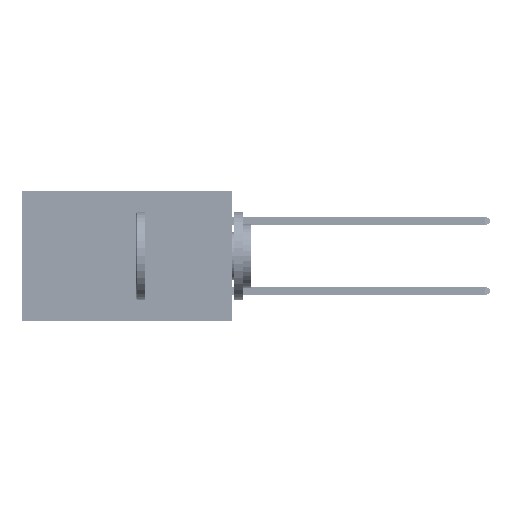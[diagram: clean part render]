
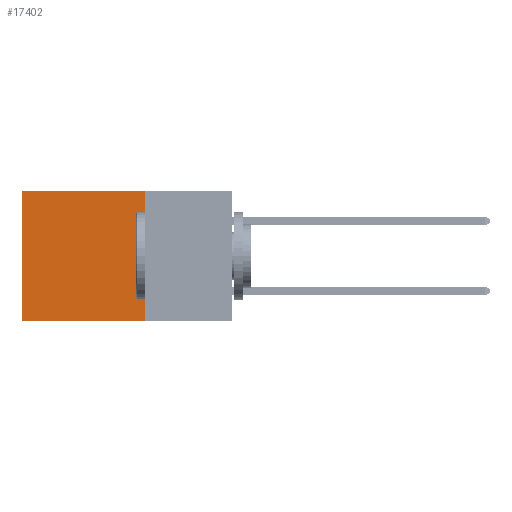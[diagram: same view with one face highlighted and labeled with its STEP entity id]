
A CAD part, left-side view. The second image highlights one B-rep face of the part: STEP entity #17402.
In plain terms, the highlighted planar face has unit normal (-1, 0, 0).
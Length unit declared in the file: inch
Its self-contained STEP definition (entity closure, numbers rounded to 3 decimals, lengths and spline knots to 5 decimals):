
#443 = VERTEX_POINT ( 'NONE', #15198 ) ;
#3101 = LINE ( 'NONE', #31345, #43478 ) ;
#3778 = EDGE_CURVE ( 'NONE', #43438, #443, #34438, .T. ) ;
#4006 = CARTESIAN_POINT ( 'NONE',  ( 0.2875, 0.25, 0. ) ) ;
#5733 = ORIENTED_EDGE ( 'NONE', *, *, #9166, .F. ) ;
#7091 = DIRECTION ( 'NONE',  ( 0., 0., -1. ) ) ;
#7413 = EDGE_LOOP ( 'NONE', ( #15483, #46881, #5733, #49461 ) ) ;
#8195 = DIRECTION ( 'NONE',  ( 0., 1., 0. ) ) ;
#8433 = FACE_OUTER_BOUND ( 'NONE', #7413, .T. ) ;
#8501 = LINE ( 'NONE', #18875, #17659 ) ;
#9166 = EDGE_CURVE ( 'NONE', #41874, #43438, #8501, .T. ) ;
#9631 = DIRECTION ( 'NONE',  ( 0., 0., -1. ) ) ;
#10554 = EDGE_CURVE ( 'NONE', #41874, #19570, #35393, .T. ) ;
#12280 = CARTESIAN_POINT ( 'NONE',  ( 0.2875, 0.25, -0.37 ) ) ;
#13038 = PLANE ( 'NONE',  #19139 ) ;
#15198 = CARTESIAN_POINT ( 'NONE',  ( 0.2875, 0.6, -0.37 ) ) ;
#15483 = ORIENTED_EDGE ( 'NONE', *, *, #44605, .T. ) ;
#17402 = ADVANCED_FACE ( 'NONE', ( #8433 ), #13038, .F. ) ;
#17659 = VECTOR ( 'NONE', #7091, 39.37008 ) ;
#18875 = CARTESIAN_POINT ( 'NONE',  ( 0.2875, 0.25, 0. ) ) ;
#19139 = AXIS2_PLACEMENT_3D ( 'NONE', #21249, #40453, #9631 ) ;
#19570 = VERTEX_POINT ( 'NONE', #34391 ) ;
#21249 = CARTESIAN_POINT ( 'NONE',  ( 0.2875, 0.25, 0. ) ) ;
#23160 = VECTOR ( 'NONE', #32349, 39.37008 ) ;
#23250 = DIRECTION ( 'NONE',  ( 0., 0., -1. ) ) ;
#31345 = CARTESIAN_POINT ( 'NONE',  ( 0.2875, 0.6, 0. ) ) ;
#32349 = DIRECTION ( 'NONE',  ( 0., 1., 0. ) ) ;
#32519 = CARTESIAN_POINT ( 'NONE',  ( 0.2875, 0.25, 0. ) ) ;
#34391 = CARTESIAN_POINT ( 'NONE',  ( 0.2875, 0.6, 0. ) ) ;
#34438 = LINE ( 'NONE', #12280, #42388 ) ;
#35393 = LINE ( 'NONE', #32519, #23160 ) ;
#40453 = DIRECTION ( 'NONE',  ( 1., 0., 0. ) ) ;
#41874 = VERTEX_POINT ( 'NONE', #4006 ) ;
#42388 = VECTOR ( 'NONE', #8195, 39.37008 ) ;
#42866 = CARTESIAN_POINT ( 'NONE',  ( 0.2875, 0.25, -0.37 ) ) ;
#43438 = VERTEX_POINT ( 'NONE', #42866 ) ;
#43478 = VECTOR ( 'NONE', #23250, 39.37008 ) ;
#44605 = EDGE_CURVE ( 'NONE', #19570, #443, #3101, .T. ) ;
#46881 = ORIENTED_EDGE ( 'NONE', *, *, #3778, .F. ) ;
#49461 = ORIENTED_EDGE ( 'NONE', *, *, #10554, .T. ) ;
